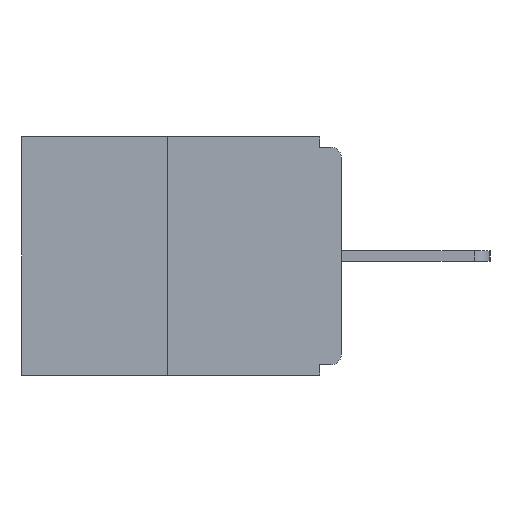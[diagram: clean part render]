
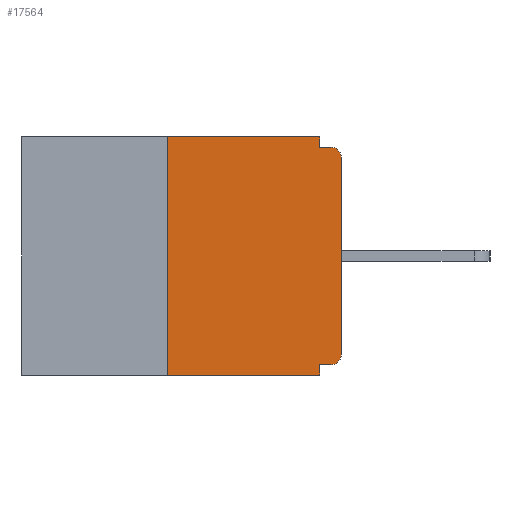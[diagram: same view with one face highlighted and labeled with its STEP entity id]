
A CAD part, left-side view. The second image highlights one B-rep face of the part: STEP entity #17564.
In plain terms, the highlighted planar face has unit normal (-1, 0, 0).
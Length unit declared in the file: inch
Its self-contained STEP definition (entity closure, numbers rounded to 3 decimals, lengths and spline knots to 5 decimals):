
#748 = VECTOR ( 'NONE', #22044, 39.37008 ) ;
#1107 = CIRCLE ( 'NONE', #7294, 0.015 ) ;
#1232 = EDGE_CURVE ( 'NONE', #13980, #21975, #6281, .T. ) ;
#1473 = DIRECTION ( 'NONE',  ( -1., 0., 0. ) ) ;
#1506 = CARTESIAN_POINT ( 'NONE',  ( 0., 0.25, -0.343 ) ) ;
#1588 = AXIS2_PLACEMENT_3D ( 'NONE', #5929, #18821, #7825 ) ;
#1857 = VERTEX_POINT ( 'NONE', #10558 ) ;
#1878 = EDGE_CURVE ( 'NONE', #8452, #20651, #2658, .T. ) ;
#2013 = PLANE ( 'NONE',  #1588 ) ;
#2252 = FACE_OUTER_BOUND ( 'NONE', #23042, .T. ) ;
#2599 = EDGE_CURVE ( 'NONE', #13980, #8452, #11437, .T. ) ;
#2658 = LINE ( 'NONE', #18526, #7698 ) ;
#2915 = EDGE_CURVE ( 'NONE', #10477, #9573, #16789, .T. ) ;
#3013 = CARTESIAN_POINT ( 'NONE',  ( 0., 0.015, -0.03 ) ) ;
#3639 = ORIENTED_EDGE ( 'NONE', *, *, #2915, .T. ) ;
#4167 = CIRCLE ( 'NONE', #4296, 0.015 ) ;
#4283 = CARTESIAN_POINT ( 'NONE',  ( 0., 0.031, -0.015 ) ) ;
#4296 = AXIS2_PLACEMENT_3D ( 'NONE', #12764, #1473, #14577 ) ;
#4420 = VERTEX_POINT ( 'NONE', #4283 ) ;
#4905 = DIRECTION ( 'NONE',  ( 0., 0., -1. ) ) ;
#5929 = CARTESIAN_POINT ( 'NONE',  ( 0., 0.46, 0. ) ) ;
#6281 = LINE ( 'NONE', #23084, #21026 ) ;
#6515 = LINE ( 'NONE', #7301, #748 ) ;
#7040 = VECTOR ( 'NONE', #13426, 39.37008 ) ;
#7053 = VECTOR ( 'NONE', #23979, 39.37008 ) ;
#7294 = AXIS2_PLACEMENT_3D ( 'NONE', #3013, #15962, #4905 ) ;
#7301 = CARTESIAN_POINT ( 'NONE',  ( 0., 0., -0.328 ) ) ;
#7615 = LINE ( 'NONE', #22627, #7040 ) ;
#7698 = VECTOR ( 'NONE', #16931, 39.37008 ) ;
#7825 = DIRECTION ( 'NONE',  ( 0., 0., -1. ) ) ;
#7986 = CARTESIAN_POINT ( 'NONE',  ( 0., 0., 0. ) ) ;
#8183 = CARTESIAN_POINT ( 'NONE',  ( 0., 0., -0.015 ) ) ;
#8452 = VERTEX_POINT ( 'NONE', #12366 ) ;
#8499 = LINE ( 'NONE', #8183, #12813 ) ;
#9573 = VERTEX_POINT ( 'NONE', #11911 ) ;
#10287 = VECTOR ( 'NONE', #11193, 39.37008 ) ;
#10477 = VERTEX_POINT ( 'NONE', #22165 ) ;
#10558 = CARTESIAN_POINT ( 'NONE',  ( 0., 0.015, -0.015 ) ) ;
#10792 = CARTESIAN_POINT ( 'NONE',  ( 0., 0.031, -0.343 ) ) ;
#11193 = DIRECTION ( 'NONE',  ( 0., 0., 1. ) ) ;
#11437 = LINE ( 'NONE', #11646, #10287 ) ;
#11552 = VERTEX_POINT ( 'NONE', #12291 ) ;
#11645 = DIRECTION ( 'NONE',  ( 0., 0., -1. ) ) ;
#11646 = CARTESIAN_POINT ( 'NONE',  ( 0., 0.25, 0. ) ) ;
#11836 = ORIENTED_EDGE ( 'NONE', *, *, #24196, .F. ) ;
#11911 = CARTESIAN_POINT ( 'NONE',  ( 0., 0., -0.03 ) ) ;
#12176 = EDGE_CURVE ( 'NONE', #9573, #1857, #1107, .T. ) ;
#12291 = CARTESIAN_POINT ( 'NONE',  ( 0., 0.015, -0.328 ) ) ;
#12366 = CARTESIAN_POINT ( 'NONE',  ( 0., 0.25, 0. ) ) ;
#12589 = CARTESIAN_POINT ( 'NONE',  ( 0., 0.031, -0.328 ) ) ;
#12764 = CARTESIAN_POINT ( 'NONE',  ( 0., 0.015, -0.313 ) ) ;
#12813 = VECTOR ( 'NONE', #19173, 39.37008 ) ;
#13426 = DIRECTION ( 'NONE',  ( 0., 0., -1. ) ) ;
#13549 = ORIENTED_EDGE ( 'NONE', *, *, #12176, .T. ) ;
#13980 = VERTEX_POINT ( 'NONE', #1506 ) ;
#14103 = ORIENTED_EDGE ( 'NONE', *, *, #17030, .F. ) ;
#14577 = DIRECTION ( 'NONE',  ( 0., 0., -1. ) ) ;
#14596 = EDGE_CURVE ( 'NONE', #11552, #10477, #4167, .T. ) ;
#15417 = VERTEX_POINT ( 'NONE', #12589 ) ;
#15483 = ORIENTED_EDGE ( 'NONE', *, *, #1878, .F. ) ;
#15962 = DIRECTION ( 'NONE',  ( -1., 0., 0. ) ) ;
#16789 = LINE ( 'NONE', #7986, #7053 ) ;
#16931 = DIRECTION ( 'NONE',  ( 0., -1., 0. ) ) ;
#17030 = EDGE_CURVE ( 'NONE', #4420, #1857, #8499, .T. ) ;
#17127 = VECTOR ( 'NONE', #11645, 39.37008 ) ;
#17564 = ADVANCED_FACE ( 'NONE', ( #2252 ), #2013, .F. ) ;
#18526 = CARTESIAN_POINT ( 'NONE',  ( 0., 0.46, 0. ) ) ;
#18821 = DIRECTION ( 'NONE',  ( 1., 0., 0. ) ) ;
#18977 = ORIENTED_EDGE ( 'NONE', *, *, #22986, .F. ) ;
#19173 = DIRECTION ( 'NONE',  ( 0., -1., 0. ) ) ;
#20437 = ORIENTED_EDGE ( 'NONE', *, *, #2599, .F. ) ;
#20651 = VERTEX_POINT ( 'NONE', #20844 ) ;
#20844 = CARTESIAN_POINT ( 'NONE',  ( 0., 0.031, 0. ) ) ;
#21026 = VECTOR ( 'NONE', #23089, 39.37008 ) ;
#21041 = ORIENTED_EDGE ( 'NONE', *, *, #1232, .T. ) ;
#21520 = LINE ( 'NONE', #22677, #17127 ) ;
#21975 = VERTEX_POINT ( 'NONE', #10792 ) ;
#22044 = DIRECTION ( 'NONE',  ( 0., 1., 0. ) ) ;
#22048 = EDGE_CURVE ( 'NONE', #11552, #15417, #6515, .T. ) ;
#22165 = CARTESIAN_POINT ( 'NONE',  ( 0., 0., -0.313 ) ) ;
#22195 = ORIENTED_EDGE ( 'NONE', *, *, #22048, .F. ) ;
#22627 = CARTESIAN_POINT ( 'NONE',  ( 0., 0.031, -0.343 ) ) ;
#22677 = CARTESIAN_POINT ( 'NONE',  ( 0., 0.031, 0. ) ) ;
#22795 = ORIENTED_EDGE ( 'NONE', *, *, #14596, .T. ) ;
#22986 = EDGE_CURVE ( 'NONE', #20651, #4420, #21520, .T. ) ;
#23042 = EDGE_LOOP ( 'NONE', ( #15483, #20437, #21041, #11836, #22195, #22795, #3639, #13549, #14103, #18977 ) ) ;
#23084 = CARTESIAN_POINT ( 'NONE',  ( 0., 0.46, -0.343 ) ) ;
#23089 = DIRECTION ( 'NONE',  ( 0., -1., 0. ) ) ;
#23979 = DIRECTION ( 'NONE',  ( 0., 0., 1. ) ) ;
#24196 = EDGE_CURVE ( 'NONE', #15417, #21975, #7615, .T. ) ;
